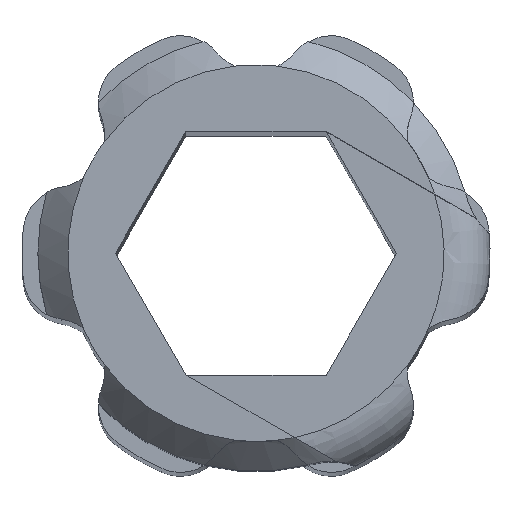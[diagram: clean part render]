
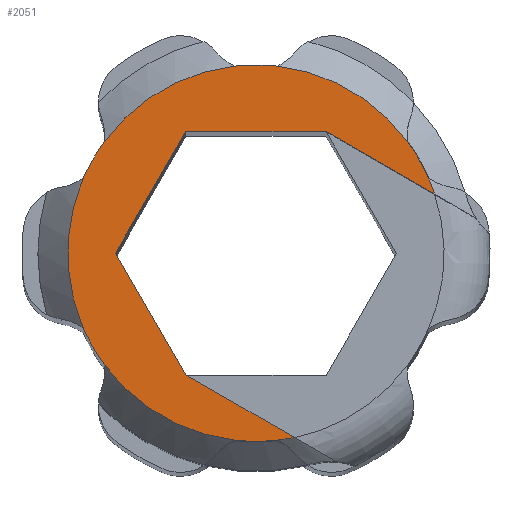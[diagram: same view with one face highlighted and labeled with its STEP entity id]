
A CAD part, top view. The second image highlights one B-rep face of the part: STEP entity #2051.
In plain terms, the highlighted planar face has unit normal (0, 0, 1).
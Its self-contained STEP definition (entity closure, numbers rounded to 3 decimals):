
#37=PLANE('',#2324);
#164=LINE('',#3469,#278);
#188=LINE('',#3706,#302);
#189=LINE('',#3753,#303);
#202=LINE('',#3837,#316);
#203=LINE('',#3838,#317);
#278=VECTOR('',#2713,10.);
#302=VECTOR('',#2849,10.);
#303=VECTOR('',#2884,10.);
#316=VECTOR('',#2951,10.);
#317=VECTOR('',#2952,10.);
#438=FACE_OUTER_BOUND('',#560,.T.);
#560=EDGE_LOOP('',(#1856,#1857,#1858,#1859,#1860,#1861,#1862,#1863,#1864,
#1865,#1866,#1867,#1868,#1869,#1870,#1871));
#694=CIRCLE('',#2178,4.1);
#709=CIRCLE('',#2213,4.1);
#737=CIRCLE('',#2264,4.1);
#740=CIRCLE('',#2273,4.1);
#742=CIRCLE('',#2279,4.1);
#753=CIRCLE('',#2301,4.1);
#754=CIRCLE('',#2305,4.1);
#755=CIRCLE('',#2308,4.1);
#757=CIRCLE('',#2317,4.1);
#758=CIRCLE('',#2321,4.1);
#759=CIRCLE('',#2323,4.1);
#832=VERTEX_POINT('',#3216);
#833=VERTEX_POINT('',#3218);
#872=VERTEX_POINT('',#3397);
#874=VERTEX_POINT('',#3408);
#887=VERTEX_POINT('',#3466);
#888=VERTEX_POINT('',#3468);
#924=VERTEX_POINT('',#3639);
#930=VERTEX_POINT('',#3683);
#931=VERTEX_POINT('',#3687);
#941=VERTEX_POINT('',#3748);
#942=VERTEX_POINT('',#3752);
#945=VERTEX_POINT('',#3765);
#946=VERTEX_POINT('',#3774);
#948=VERTEX_POINT('',#3811);
#949=VERTEX_POINT('',#3820);
#950=VERTEX_POINT('',#3836);
#1061=EDGE_CURVE('',#832,#833,#694,.T.);
#1122=EDGE_CURVE('',#874,#872,#709,.T.);
#1143=EDGE_CURVE('',#888,#887,#164,.T.);
#1189=EDGE_CURVE('',#833,#874,#737,.T.);
#1203=EDGE_CURVE('',#924,#832,#740,.T.);
#1213=EDGE_CURVE('',#930,#931,#742,.T.);
#1217=EDGE_CURVE('',#930,#888,#188,.T.);
#1232=EDGE_CURVE('',#942,#941,#189,.T.);
#1240=EDGE_CURVE('',#946,#945,#753,.T.);
#1243=EDGE_CURVE('',#931,#924,#754,.T.);
#1245=EDGE_CURVE('',#945,#941,#755,.T.);
#1254=EDGE_CURVE('',#948,#949,#757,.T.);
#1257=EDGE_CURVE('',#949,#946,#758,.T.);
#1258=EDGE_CURVE('',#872,#948,#759,.T.);
#1259=EDGE_CURVE('',#887,#950,#202,.T.);
#1260=EDGE_CURVE('',#950,#942,#203,.T.);
#1856=ORIENTED_EDGE('',*,*,#1213,.F.);
#1857=ORIENTED_EDGE('',*,*,#1217,.T.);
#1858=ORIENTED_EDGE('',*,*,#1143,.T.);
#1859=ORIENTED_EDGE('',*,*,#1259,.T.);
#1860=ORIENTED_EDGE('',*,*,#1260,.T.);
#1861=ORIENTED_EDGE('',*,*,#1232,.T.);
#1862=ORIENTED_EDGE('',*,*,#1245,.F.);
#1863=ORIENTED_EDGE('',*,*,#1240,.F.);
#1864=ORIENTED_EDGE('',*,*,#1257,.F.);
#1865=ORIENTED_EDGE('',*,*,#1254,.F.);
#1866=ORIENTED_EDGE('',*,*,#1258,.F.);
#1867=ORIENTED_EDGE('',*,*,#1122,.F.);
#1868=ORIENTED_EDGE('',*,*,#1189,.F.);
#1869=ORIENTED_EDGE('',*,*,#1061,.F.);
#1870=ORIENTED_EDGE('',*,*,#1203,.F.);
#1871=ORIENTED_EDGE('',*,*,#1243,.F.);
#2051=ADVANCED_FACE('',(#438),#37,.T.);
#2178=AXIS2_PLACEMENT_3D('',#3219,#2573,#2574);
#2213=AXIS2_PLACEMENT_3D('',#3410,#2676,#2677);
#2264=AXIS2_PLACEMENT_3D('',#3590,#2808,#2809);
#2273=AXIS2_PLACEMENT_3D('',#3646,#2830,#2831);
#2279=AXIS2_PLACEMENT_3D('',#3688,#2844,#2845);
#2301=AXIS2_PLACEMENT_3D('',#3776,#2896,#2897);
#2305=AXIS2_PLACEMENT_3D('',#3787,#2905,#2906);
#2308=AXIS2_PLACEMENT_3D('',#3791,#2912,#2913);
#2317=AXIS2_PLACEMENT_3D('',#3821,#2934,#2935);
#2321=AXIS2_PLACEMENT_3D('',#3832,#2943,#2944);
#2323=AXIS2_PLACEMENT_3D('',#3834,#2947,#2948);
#2324=AXIS2_PLACEMENT_3D('',#3835,#2949,#2950);
#2573=DIRECTION('center_axis',(0.,0.,
-1.));
#2574=DIRECTION('ref_axis',(-1.,0.,0.));
#2676=DIRECTION('center_axis',(0.,0.,
-1.));
#2677=DIRECTION('ref_axis',(-1.,0.,0.));
#2713=DIRECTION('',(-0.5,0.866,0.));
#2808=DIRECTION('center_axis',(0.,0.,
-1.));
#2809=DIRECTION('ref_axis',(-1.,0.,0.));
#2830=DIRECTION('center_axis',(0.,0.,
-1.));
#2831=DIRECTION('ref_axis',(-1.,0.,0.));
#2844=DIRECTION('center_axis',(0.,0.,
-1.));
#2845=DIRECTION('ref_axis',(-1.,0.,0.));
#2849=DIRECTION('',(-0.866,0.5,0.));
#2884=DIRECTION('',(0.866,-0.5,0.));
#2896=DIRECTION('center_axis',(0.,0.,
-1.));
#2897=DIRECTION('ref_axis',(-1.,0.,0.));
#2905=DIRECTION('center_axis',(0.,0.,
-1.));
#2906=DIRECTION('ref_axis',(-1.,0.,0.));
#2912=DIRECTION('center_axis',(0.,0.,
-1.));
#2913=DIRECTION('ref_axis',(-1.,0.,0.));
#2934=DIRECTION('center_axis',(0.,0.,
-1.));
#2935=DIRECTION('ref_axis',(-1.,0.,0.));
#2943=DIRECTION('center_axis',(0.,0.,
-1.));
#2944=DIRECTION('ref_axis',(-1.,0.,0.));
#2947=DIRECTION('center_axis',(0.,0.,
-1.));
#2948=DIRECTION('ref_axis',(-1.,0.,0.));
#2949=DIRECTION('center_axis',(0.,0.,
1.));
#2950=DIRECTION('ref_axis',(0.5,0.866,0.));
#2951=DIRECTION('',(0.5,0.866,0.));
#2952=DIRECTION('',(1.,0.,0.));
#3216=CARTESIAN_POINT('',(-3.297,33.033,41.47));
#3218=CARTESIAN_POINT('',(-3.759,33.833,41.47));
#3219=CARTESIAN_POINT('Origin',(0.,35.47,41.47));
#3397=CARTESIAN_POINT('',(-3.297,37.907,41.47));
#3408=CARTESIAN_POINT('',(-3.759,37.107,41.47));
#3410=CARTESIAN_POINT('Origin',(0.,35.47,41.47));
#3466=CARTESIAN_POINT('',(-3.06,35.47,41.47));
#3468=CARTESIAN_POINT('',(-1.53,32.82,41.47));
#3469=CARTESIAN_POINT('',(-1.53,32.82,41.47));
#3590=CARTESIAN_POINT('Origin',(0.,35.47,41.47));
#3639=CARTESIAN_POINT('',(-0.461,31.396,41.47));
#3646=CARTESIAN_POINT('Origin',(0.,35.47,41.47));
#3683=CARTESIAN_POINT('',(0.833,31.456,41.47));
#3687=CARTESIAN_POINT('',(0.461,31.396,41.47));
#3688=CARTESIAN_POINT('Origin',(0.,35.47,41.47));
#3706=CARTESIAN_POINT('',(-1.53,32.82,41.47));
#3748=CARTESIAN_POINT('',(3.893,36.756,41.47));
#3752=CARTESIAN_POINT('',(1.53,38.12,41.47));
#3753=CARTESIAN_POINT('',(1.53,38.12,41.47));
#3765=CARTESIAN_POINT('',(3.759,37.107,41.47));
#3774=CARTESIAN_POINT('',(3.297,37.907,41.47));
#3776=CARTESIAN_POINT('Origin',(0.,35.47,41.47));
#3787=CARTESIAN_POINT('Origin',(0.,35.47,41.47));
#3791=CARTESIAN_POINT('Origin',(0.,35.47,41.47));
#3811=CARTESIAN_POINT('',(-0.461,39.544,41.47));
#3820=CARTESIAN_POINT('',(0.461,39.544,41.47));
#3821=CARTESIAN_POINT('Origin',(0.,35.47,41.47));
#3832=CARTESIAN_POINT('Origin',(0.,35.47,41.47));
#3834=CARTESIAN_POINT('Origin',(0.,35.47,41.47));
#3835=CARTESIAN_POINT('Origin',(0.,35.47,
41.47));
#3836=CARTESIAN_POINT('',(-1.53,38.12,41.47));
#3837=CARTESIAN_POINT('',(-3.06,35.47,41.47));
#3838=CARTESIAN_POINT('',(-1.53,38.12,41.47));
